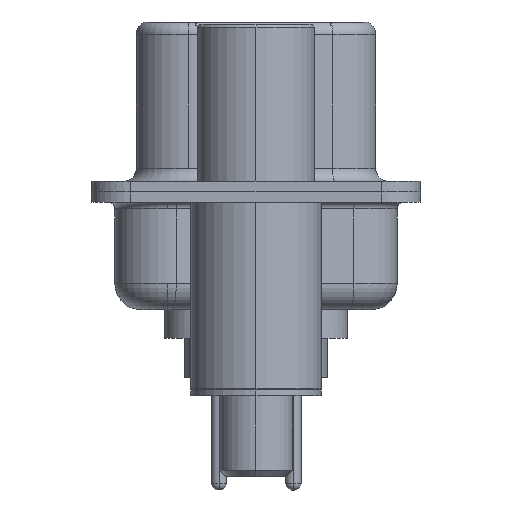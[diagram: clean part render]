
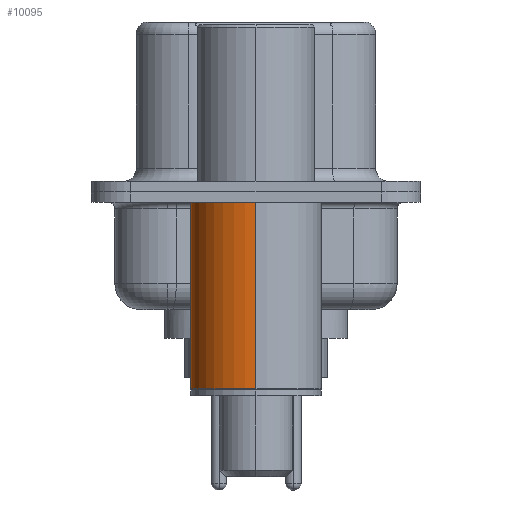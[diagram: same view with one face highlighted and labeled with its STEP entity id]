
A CAD part, left-side view. The second image highlights one B-rep face of the part: STEP entity #10095.
In plain terms, the highlighted cylindrical face has radius 2.5 mm (diameter 5 mm), a partial arc.
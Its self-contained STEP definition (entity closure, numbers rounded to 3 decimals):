
#1054 = CIRCLE ( 'NONE', #5118, 2.5 ) ;
#1143 = EDGE_CURVE ( 'NONE', #1460, #5171, #1054, .T. ) ;
#1460 = VERTEX_POINT ( 'NONE', #9373 ) ;
#1597 = VECTOR ( 'NONE', #19885, 1000. ) ;
#2841 = ORIENTED_EDGE ( 'NONE', *, *, #11133, .F. ) ;
#3787 = EDGE_CURVE ( 'NONE', #14907, #12357, #16625, .T. ) ;
#4354 = DIRECTION ( 'NONE',  ( 1., 0., 0. ) ) ;
#5088 = DIRECTION ( 'NONE',  ( 1., 0., 0. ) ) ;
#5118 = AXIS2_PLACEMENT_3D ( 'NONE', #15895, #15723, #5088 ) ;
#5171 = VERTEX_POINT ( 'NONE', #8642 ) ;
#5338 = ORIENTED_EDGE ( 'NONE', *, *, #1143, .F. ) ;
#5839 = AXIS2_PLACEMENT_3D ( 'NONE', #6471, #9697, #17753 ) ;
#6471 = CARTESIAN_POINT ( 'NONE',  ( 0., 0., 0.581 ) ) ;
#7813 = CARTESIAN_POINT ( 'NONE',  ( -2.5, 0., -7.525 ) ) ;
#8642 = CARTESIAN_POINT ( 'NONE',  ( -2.5, 0., -0.4 ) ) ;
#9373 = CARTESIAN_POINT ( 'NONE',  ( 2.5, 0., -0.4 ) ) ;
#9697 = DIRECTION ( 'NONE',  ( 0., 0., 1. ) ) ;
#9787 = EDGE_LOOP ( 'NONE', ( #13747, #20337, #5338, #2841 ) ) ;
#10095 = ADVANCED_FACE ( 'NONE', ( #19198 ), #10725, .T. ) ;
#10398 = LINE ( 'NONE', #16045, #18405 ) ;
#10725 = CYLINDRICAL_SURFACE ( 'NONE', #5839, 2.5 ) ;
#11133 = EDGE_CURVE ( 'NONE', #14907, #1460, #17908, .T. ) ;
#11403 = CARTESIAN_POINT ( 'NONE',  ( 2.5, 0., -7.525 ) ) ;
#11496 = EDGE_CURVE ( 'NONE', #12357, #5171, #10398, .T. ) ;
#12357 = VERTEX_POINT ( 'NONE', #7813 ) ;
#12848 = DIRECTION ( 'NONE',  ( 0., 0., 1. ) ) ;
#13747 = ORIENTED_EDGE ( 'NONE', *, *, #3787, .T. ) ;
#14907 = VERTEX_POINT ( 'NONE', #11403 ) ;
#15085 = CARTESIAN_POINT ( 'NONE',  ( 2.5, 0., 0.581 ) ) ;
#15192 = AXIS2_PLACEMENT_3D ( 'NONE', #17470, #20473, #4354 ) ;
#15723 = DIRECTION ( 'NONE',  ( 0., 0., 1. ) ) ;
#15895 = CARTESIAN_POINT ( 'NONE',  ( 0., 0., -0.4 ) ) ;
#16045 = CARTESIAN_POINT ( 'NONE',  ( -2.5, 0., 0.581 ) ) ;
#16625 = CIRCLE ( 'NONE', #15192, 2.5 ) ;
#17470 = CARTESIAN_POINT ( 'NONE',  ( 0., 0., -7.525 ) ) ;
#17753 = DIRECTION ( 'NONE',  ( 1., 0., 0. ) ) ;
#17908 = LINE ( 'NONE', #15085, #1597 ) ;
#18405 = VECTOR ( 'NONE', #12848, 1000. ) ;
#19198 = FACE_OUTER_BOUND ( 'NONE', #9787, .T. ) ;
#19885 = DIRECTION ( 'NONE',  ( 0., 0., 1. ) ) ;
#20337 = ORIENTED_EDGE ( 'NONE', *, *, #11496, .T. ) ;
#20473 = DIRECTION ( 'NONE',  ( 0., 0., 1. ) ) ;
